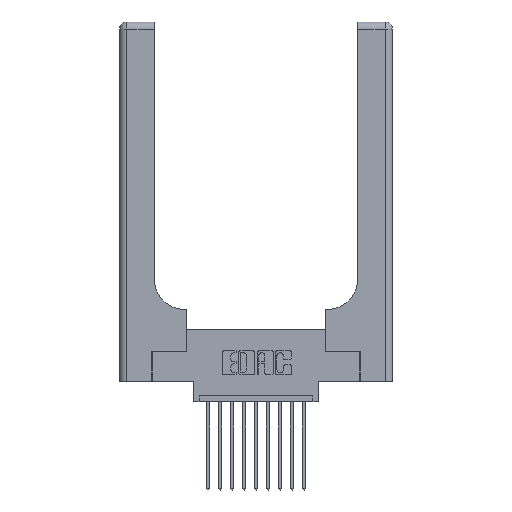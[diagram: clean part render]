
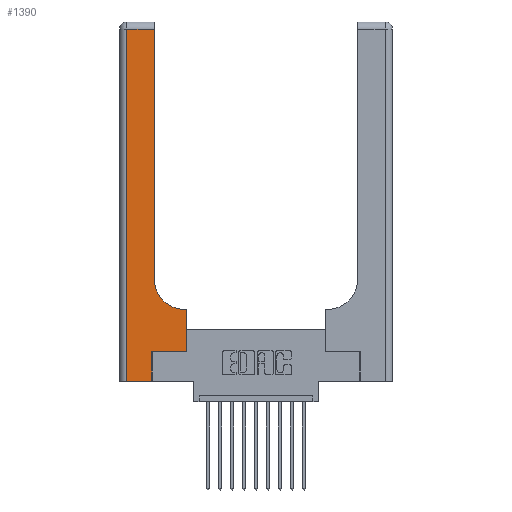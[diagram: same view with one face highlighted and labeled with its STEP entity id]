
A CAD part, top view. The second image highlights one B-rep face of the part: STEP entity #1390.
In plain terms, the highlighted planar face has unit normal (0, 0, 1).
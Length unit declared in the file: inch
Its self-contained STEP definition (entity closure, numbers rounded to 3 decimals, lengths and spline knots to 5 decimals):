
#180 = VERTEX_POINT ( 'NONE', #4604 ) ;
#485 = LINE ( 'NONE', #7931, #2285 ) ;
#896 = LINE ( 'NONE', #10145, #2129 ) ;
#1150 = DIRECTION ( 'NONE',  ( -1., 0., 0. ) ) ;
#1298 = LINE ( 'NONE', #5350, #6507 ) ;
#1390 = ADVANCED_FACE ( 'NONE', ( #4750 ), #4461, .F. ) ;
#1602 = VECTOR ( 'NONE', #15842, 39.37008 ) ;
#1774 = CARTESIAN_POINT ( 'NONE',  ( 0.269, 0., 0.37 ) ) ;
#1796 = CARTESIAN_POINT ( 'NONE',  ( 0.2915, 0.85, 0.37 ) ) ;
#1955 = LINE ( 'NONE', #3351, #2722 ) ;
#2018 = CARTESIAN_POINT ( 'NONE',  ( 0., 3., 0.37 ) ) ;
#2129 = VECTOR ( 'NONE', #10096, 39.37008 ) ;
#2285 = VECTOR ( 'NONE', #16130, 39.37008 ) ;
#2483 = EDGE_CURVE ( 'NONE', #7698, #16469, #1298, .T. ) ;
#2542 = VERTEX_POINT ( 'NONE', #12759 ) ;
#2722 = VECTOR ( 'NONE', #5747, 39.37008 ) ;
#3351 = CARTESIAN_POINT ( 'NONE',  ( 0.2915, 0.6, 0.37 ) ) ;
#3356 = DIRECTION ( 'NONE',  ( 0., -1., 0. ) ) ;
#3428 = EDGE_CURVE ( 'NONE', #16469, #2542, #485, .T. ) ;
#3468 = VECTOR ( 'NONE', #3356, 39.37008 ) ;
#3475 = CARTESIAN_POINT ( 'NONE',  ( 0.269, 0.25, 0.37 ) ) ;
#3630 = CARTESIAN_POINT ( 'NONE',  ( 0.5415, 0.6, 0.37 ) ) ;
#3769 = EDGE_CURVE ( 'NONE', #9808, #180, #14663, .T. ) ;
#3860 = AXIS2_PLACEMENT_3D ( 'NONE', #14581, #10691, #13161 ) ;
#4461 = PLANE ( 'NONE',  #5733 ) ;
#4604 = CARTESIAN_POINT ( 'NONE',  ( 0.06, 0., 0.37 ) ) ;
#4750 = FACE_OUTER_BOUND ( 'NONE', #7584, .T. ) ;
#4977 = LINE ( 'NONE', #1774, #1602 ) ;
#5292 = DIRECTION ( 'NONE',  ( 1., 0., 0. ) ) ;
#5350 = CARTESIAN_POINT ( 'NONE',  ( 0.269, 0.25, 0.37 ) ) ;
#5558 = CARTESIAN_POINT ( 'NONE',  ( 0.5585, 0.25, 0.37 ) ) ;
#5733 = AXIS2_PLACEMENT_3D ( 'NONE', #2018, #14745, #11958 ) ;
#5747 = DIRECTION ( 'NONE',  ( -1., 0., 0. ) ) ;
#5986 = VERTEX_POINT ( 'NONE', #8558 ) ;
#6069 = CARTESIAN_POINT ( 'NONE',  ( 0.06, 2.94, 0.37 ) ) ;
#6507 = VECTOR ( 'NONE', #5292, 39.37008 ) ;
#6800 = EDGE_CURVE ( 'NONE', #5986, #7698, #4977, .T. ) ;
#6944 = ORIENTED_EDGE ( 'NONE', *, *, #2483, .T. ) ;
#7021 = ORIENTED_EDGE ( 'NONE', *, *, #3769, .T. ) ;
#7498 = CIRCLE ( 'NONE', #3860, 0.25 ) ;
#7584 = EDGE_LOOP ( 'NONE', ( #8707, #8602, #7021, #12293, #7607, #6944, #10551, #16009, #12968 ) ) ;
#7607 = ORIENTED_EDGE ( 'NONE', *, *, #6800, .T. ) ;
#7698 = VERTEX_POINT ( 'NONE', #3475 ) ;
#7931 = CARTESIAN_POINT ( 'NONE',  ( 0.5585, 0.25, 0.37 ) ) ;
#8558 = CARTESIAN_POINT ( 'NONE',  ( 0.269, 0., 0.37 ) ) ;
#8602 = ORIENTED_EDGE ( 'NONE', *, *, #12229, .T. ) ;
#8707 = ORIENTED_EDGE ( 'NONE', *, *, #15334, .T. ) ;
#9295 = VECTOR ( 'NONE', #12485, 39.37008 ) ;
#9650 = EDGE_CURVE ( 'NONE', #10971, #14299, #7498, .T. ) ;
#9808 = VERTEX_POINT ( 'NONE', #6069 ) ;
#10096 = DIRECTION ( 'NONE',  ( 1., 0., 0. ) ) ;
#10145 = CARTESIAN_POINT ( 'NONE',  ( 0., 0., 0.37 ) ) ;
#10551 = ORIENTED_EDGE ( 'NONE', *, *, #3428, .T. ) ;
#10691 = DIRECTION ( 'NONE',  ( 0., 0., -1. ) ) ;
#10803 = CARTESIAN_POINT ( 'NONE',  ( 0.06, 3., 0.37 ) ) ;
#10945 = VERTEX_POINT ( 'NONE', #15204 ) ;
#10971 = VERTEX_POINT ( 'NONE', #3630 ) ;
#11138 = CARTESIAN_POINT ( 'NONE',  ( 0.2915, 3., 0.37 ) ) ;
#11958 = DIRECTION ( 'NONE',  ( -1., 0., 0. ) ) ;
#12229 = EDGE_CURVE ( 'NONE', #10945, #9808, #12367, .T. ) ;
#12293 = ORIENTED_EDGE ( 'NONE', *, *, #15449, .T. ) ;
#12367 = LINE ( 'NONE', #12705, #15011 ) ;
#12485 = DIRECTION ( 'NONE',  ( 0., 1., 0. ) ) ;
#12705 = CARTESIAN_POINT ( 'NONE',  ( 0., 2.94, 0.37 ) ) ;
#12759 = CARTESIAN_POINT ( 'NONE',  ( 0.5585, 0.6, 0.37 ) ) ;
#12968 = ORIENTED_EDGE ( 'NONE', *, *, #9650, .T. ) ;
#13161 = DIRECTION ( 'NONE',  ( 1., 0., 0. ) ) ;
#14299 = VERTEX_POINT ( 'NONE', #1796 ) ;
#14518 = EDGE_CURVE ( 'NONE', #2542, #10971, #1955, .T. ) ;
#14581 = CARTESIAN_POINT ( 'NONE',  ( 0.5415, 0.85, 0.37 ) ) ;
#14663 = LINE ( 'NONE', #10803, #3468 ) ;
#14745 = DIRECTION ( 'NONE',  ( 0., 0., -1. ) ) ;
#15011 = VECTOR ( 'NONE', #1150, 39.37008 ) ;
#15204 = CARTESIAN_POINT ( 'NONE',  ( 0.2915, 2.94, 0.37 ) ) ;
#15334 = EDGE_CURVE ( 'NONE', #14299, #10945, #16294, .T. ) ;
#15449 = EDGE_CURVE ( 'NONE', #180, #5986, #896, .T. ) ;
#15842 = DIRECTION ( 'NONE',  ( 0., 1., 0. ) ) ;
#16009 = ORIENTED_EDGE ( 'NONE', *, *, #14518, .T. ) ;
#16130 = DIRECTION ( 'NONE',  ( 0., 1., 0. ) ) ;
#16294 = LINE ( 'NONE', #11138, #9295 ) ;
#16469 = VERTEX_POINT ( 'NONE', #5558 ) ;
